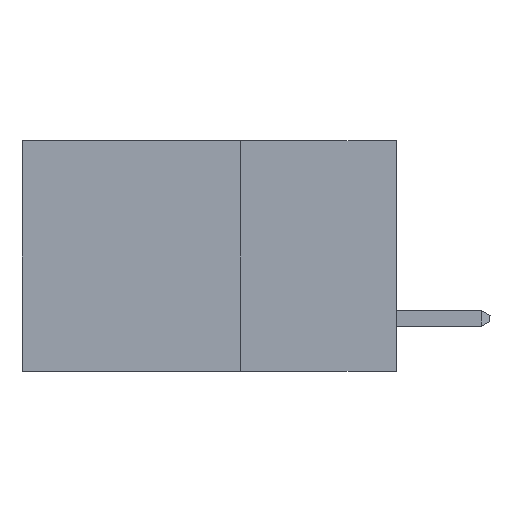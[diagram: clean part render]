
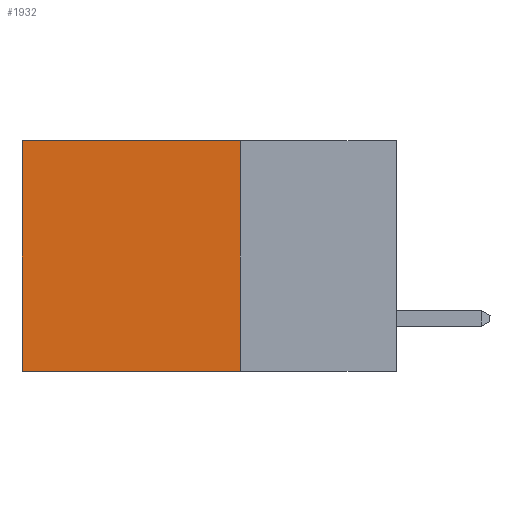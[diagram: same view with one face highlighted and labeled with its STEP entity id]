
A CAD part, left-side view. The second image highlights one B-rep face of the part: STEP entity #1932.
In plain terms, the highlighted planar face has unit normal (-1, 0, 0).
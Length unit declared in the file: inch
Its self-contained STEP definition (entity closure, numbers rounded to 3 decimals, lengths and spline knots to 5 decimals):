
#39 = CARTESIAN_POINT ( 'NONE',  ( 0.2615, 0.25, -0.37 ) ) ;
#69 = EDGE_CURVE ( 'NONE', #4880, #10406, #1247, .T. ) ;
#213 = DIRECTION ( 'NONE',  ( 0., 0., -1. ) ) ;
#595 = LINE ( 'NONE', #8333, #3266 ) ;
#634 = EDGE_CURVE ( 'NONE', #3574, #4265, #7220, .T. ) ;
#861 = DIRECTION ( 'NONE',  ( 1., 0., 0. ) ) ;
#1247 = LINE ( 'NONE', #1673, #9995 ) ;
#1673 = CARTESIAN_POINT ( 'NONE',  ( 0.2615, 0.25, -0.37 ) ) ;
#1892 = CARTESIAN_POINT ( 'NONE',  ( 0.2615, 0.25, -0.37 ) ) ;
#1932 = ADVANCED_FACE ( 'NONE', ( #1936 ), #3863, .F. ) ;
#1936 = FACE_OUTER_BOUND ( 'NONE', #5335, .T. ) ;
#2503 = VECTOR ( 'NONE', #2618, 39.37008 ) ;
#2618 = DIRECTION ( 'NONE',  ( 0., 1., 0. ) ) ;
#2735 = EDGE_CURVE ( 'NONE', #10406, #4265, #9384, .T. ) ;
#3266 = VECTOR ( 'NONE', #8505, 39.37008 ) ;
#3574 = VERTEX_POINT ( 'NONE', #4056 ) ;
#3863 = PLANE ( 'NONE',  #8049 ) ;
#3942 = DIRECTION ( 'NONE',  ( 0., 0., -1. ) ) ;
#4056 = CARTESIAN_POINT ( 'NONE',  ( 0.2615, 0.6, 0. ) ) ;
#4265 = VERTEX_POINT ( 'NONE', #8799 ) ;
#4316 = ORIENTED_EDGE ( 'NONE', *, *, #634, .T. ) ;
#4324 = ORIENTED_EDGE ( 'NONE', *, *, #2735, .F. ) ;
#4358 = ORIENTED_EDGE ( 'NONE', *, *, #69, .F. ) ;
#4368 = ORIENTED_EDGE ( 'NONE', *, *, #6758, .T. ) ;
#4880 = VERTEX_POINT ( 'NONE', #9429 ) ;
#5335 = EDGE_LOOP ( 'NONE', ( #4316, #4324, #4358, #4368 ) ) ;
#6758 = EDGE_CURVE ( 'NONE', #4880, #3574, #595, .T. ) ;
#7095 = DIRECTION ( 'NONE',  ( 0., 0., -1. ) ) ;
#7220 = LINE ( 'NONE', #8460, #10661 ) ;
#8049 = AXIS2_PLACEMENT_3D ( 'NONE', #1892, #861, #3942 ) ;
#8333 = CARTESIAN_POINT ( 'NONE',  ( 0.2615, 0.25, 0. ) ) ;
#8460 = CARTESIAN_POINT ( 'NONE',  ( 0.2615, 0.6, -0.37 ) ) ;
#8505 = DIRECTION ( 'NONE',  ( 0., 1., 0. ) ) ;
#8799 = CARTESIAN_POINT ( 'NONE',  ( 0.2615, 0.6, -0.37 ) ) ;
#9384 = LINE ( 'NONE', #39, #2503 ) ;
#9429 = CARTESIAN_POINT ( 'NONE',  ( 0.2615, 0.25, 0. ) ) ;
#9995 = VECTOR ( 'NONE', #213, 39.37008 ) ;
#10221 = CARTESIAN_POINT ( 'NONE',  ( 0.2615, 0.25, -0.37 ) ) ;
#10406 = VERTEX_POINT ( 'NONE', #10221 ) ;
#10661 = VECTOR ( 'NONE', #7095, 39.37008 ) ;
